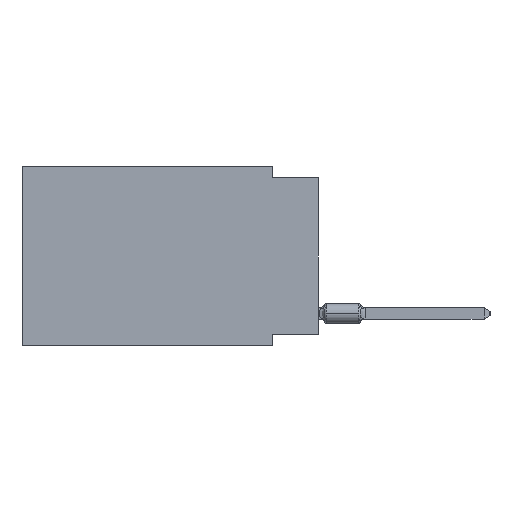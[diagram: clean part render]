
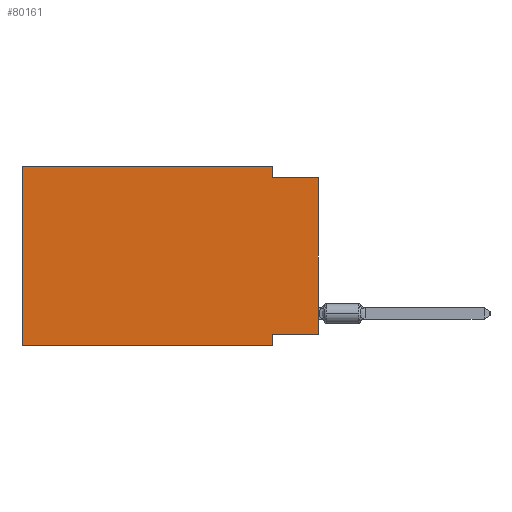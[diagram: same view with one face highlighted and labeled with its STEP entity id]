
A CAD part, left-side view. The second image highlights one B-rep face of the part: STEP entity #80161.
In plain terms, the highlighted planar face has unit normal (-1, 0, 0).
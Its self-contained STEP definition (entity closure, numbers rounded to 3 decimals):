
#1913 = ORIENTED_EDGE ( 'NONE', *, *, #61057, .F. ) ;
#3779 = CARTESIAN_POINT ( 'NONE',  ( 0., 0., -9.271 ) ) ;
#4392 = DIRECTION ( 'NONE',  ( 0., -1., 0. ) ) ;
#5058 = DIRECTION ( 'NONE',  ( 0., -1., 0. ) ) ;
#5987 = VERTEX_POINT ( 'NONE', #20166 ) ;
#6872 = FACE_OUTER_BOUND ( 'NONE', #22852, .T. ) ;
#9780 = LINE ( 'NONE', #16895, #86329 ) ;
#11162 = DIRECTION ( 'NONE',  ( 0., 0., -1. ) ) ;
#11422 = LINE ( 'NONE', #51132, #50779 ) ;
#12506 = LINE ( 'NONE', #45929, #41609 ) ;
#13592 = CARTESIAN_POINT ( 'NONE',  ( 0., 2.54, -9.271 ) ) ;
#14703 = CARTESIAN_POINT ( 'NONE',  ( 0., 0., -9.271 ) ) ;
#15073 = EDGE_CURVE ( 'NONE', #77373, #75914, #82480, .T. ) ;
#16895 = CARTESIAN_POINT ( 'NONE',  ( 0., 0., 0. ) ) ;
#19475 = EDGE_CURVE ( 'NONE', #86735, #43933, #12506, .T. ) ;
#20166 = CARTESIAN_POINT ( 'NONE',  ( 0., 2.54, -9.906 ) ) ;
#20794 = CARTESIAN_POINT ( 'NONE',  ( 0., 2.54, -9.906 ) ) ;
#22852 = EDGE_LOOP ( 'NONE', ( #63202, #85413, #1913, #32832, #80386, #30543, #64007, #35385 ) ) ;
#24375 = VERTEX_POINT ( 'NONE', #38627 ) ;
#25334 = CARTESIAN_POINT ( 'NONE',  ( 0., 2.54, -0.635 ) ) ;
#30543 = ORIENTED_EDGE ( 'NONE', *, *, #84315, .T. ) ;
#32832 = ORIENTED_EDGE ( 'NONE', *, *, #19475, .F. ) ;
#33453 = VERTEX_POINT ( 'NONE', #53148 ) ;
#33822 = VECTOR ( 'NONE', #79174, 1000. ) ;
#33907 = DIRECTION ( 'NONE',  ( 0., 1., 0. ) ) ;
#34021 = PLANE ( 'NONE',  #40820 ) ;
#35385 = ORIENTED_EDGE ( 'NONE', *, *, #15073, .F. ) ;
#36855 = EDGE_CURVE ( 'NONE', #75470, #24375, #38235, .T. ) ;
#38235 = LINE ( 'NONE', #46239, #60377 ) ;
#38627 = CARTESIAN_POINT ( 'NONE',  ( 0., 0., -0.635 ) ) ;
#40820 = AXIS2_PLACEMENT_3D ( 'NONE', #61231, #61657, #58715 ) ;
#41465 = EDGE_CURVE ( 'NONE', #77373, #24375, #9780, .T. ) ;
#41609 = VECTOR ( 'NONE', #46821, 1000. ) ;
#42640 = VECTOR ( 'NONE', #33907, 1000. ) ;
#43933 = VERTEX_POINT ( 'NONE', #63753 ) ;
#45929 = CARTESIAN_POINT ( 'NONE',  ( 0., 16.383, 0. ) ) ;
#46239 = CARTESIAN_POINT ( 'NONE',  ( 0., 0., -0.635 ) ) ;
#46821 = DIRECTION ( 'NONE',  ( 0., -1., 0. ) ) ;
#50779 = VECTOR ( 'NONE', #78754, 1000. ) ;
#51132 = CARTESIAN_POINT ( 'NONE',  ( 0., 16.383, 0. ) ) ;
#53148 = CARTESIAN_POINT ( 'NONE',  ( 0., 16.383, -9.906 ) ) ;
#58670 = LINE ( 'NONE', #72912, #33822 ) ;
#58715 = DIRECTION ( 'NONE',  ( 0., 0., -1. ) ) ;
#60377 = VECTOR ( 'NONE', #4392, 1000. ) ;
#61002 = VECTOR ( 'NONE', #11162, 1000. ) ;
#61057 = EDGE_CURVE ( 'NONE', #43933, #75470, #58670, .T. ) ;
#61231 = CARTESIAN_POINT ( 'NONE',  ( 0., 16.383, 0. ) ) ;
#61657 = DIRECTION ( 'NONE',  ( 1., 0., 0. ) ) ;
#63202 = ORIENTED_EDGE ( 'NONE', *, *, #41465, .T. ) ;
#63538 = EDGE_CURVE ( 'NONE', #75914, #5987, #86916, .T. ) ;
#63753 = CARTESIAN_POINT ( 'NONE',  ( 0., 2.54, 0. ) ) ;
#64007 = ORIENTED_EDGE ( 'NONE', *, *, #63538, .F. ) ;
#68329 = CARTESIAN_POINT ( 'NONE',  ( 0., 16.383, 0. ) ) ;
#70400 = DIRECTION ( 'NONE',  ( 0., 0., 1. ) ) ;
#72912 = CARTESIAN_POINT ( 'NONE',  ( 0., 2.54, 0. ) ) ;
#75470 = VERTEX_POINT ( 'NONE', #25334 ) ;
#75914 = VERTEX_POINT ( 'NONE', #13592 ) ;
#77373 = VERTEX_POINT ( 'NONE', #3779 ) ;
#78347 = EDGE_CURVE ( 'NONE', #33453, #86735, #11422, .T. ) ;
#78705 = VECTOR ( 'NONE', #5058, 1000. ) ;
#78754 = DIRECTION ( 'NONE',  ( 0., 0., 1. ) ) ;
#79174 = DIRECTION ( 'NONE',  ( 0., 0., -1. ) ) ;
#80161 = ADVANCED_FACE ( 'NONE', ( #6872 ), #34021, .F. ) ;
#80386 = ORIENTED_EDGE ( 'NONE', *, *, #78347, .F. ) ;
#82480 = LINE ( 'NONE', #14703, #42640 ) ;
#84315 = EDGE_CURVE ( 'NONE', #33453, #5987, #86165, .T. ) ;
#85413 = ORIENTED_EDGE ( 'NONE', *, *, #36855, .F. ) ;
#85720 = CARTESIAN_POINT ( 'NONE',  ( 0., 16.383, -9.906 ) ) ;
#86165 = LINE ( 'NONE', #85720, #78705 ) ;
#86329 = VECTOR ( 'NONE', #70400, 1000. ) ;
#86735 = VERTEX_POINT ( 'NONE', #68329 ) ;
#86916 = LINE ( 'NONE', #20794, #61002 ) ;
